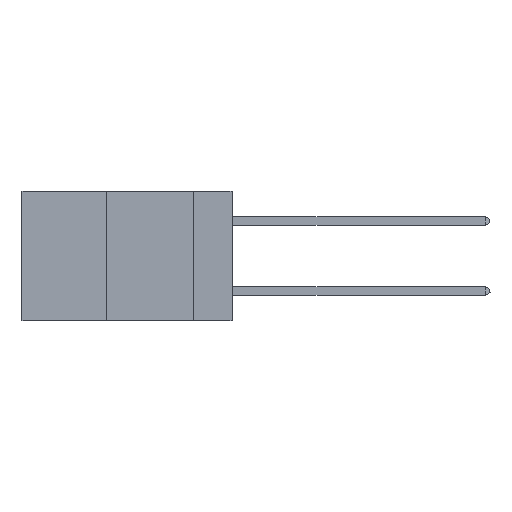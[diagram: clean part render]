
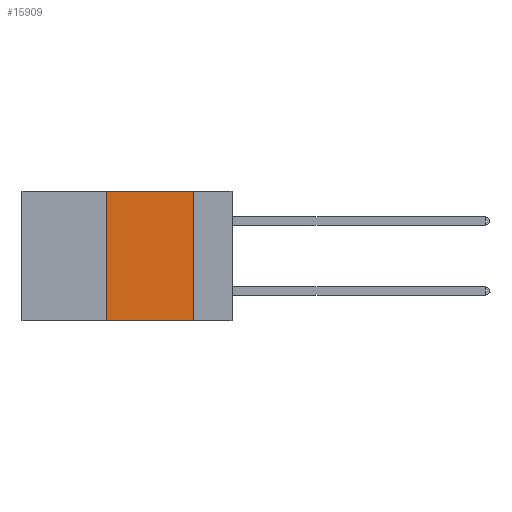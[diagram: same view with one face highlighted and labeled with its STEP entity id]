
A CAD part, left-side view. The second image highlights one B-rep face of the part: STEP entity #15909.
In plain terms, the highlighted planar face has unit normal (-1, 0, 0).
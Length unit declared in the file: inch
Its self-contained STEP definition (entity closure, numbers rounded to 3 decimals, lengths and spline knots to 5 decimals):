
#250 = VECTOR ( 'NONE', #10562, 39.37008 ) ;
#861 = ORIENTED_EDGE ( 'NONE', *, *, #14837, .F. ) ;
#1479 = EDGE_CURVE ( 'NONE', #26669, #21563, #15591, .T. ) ;
#1637 = DIRECTION ( 'NONE',  ( 0., 0., -1. ) ) ;
#2189 = CARTESIAN_POINT ( 'NONE',  ( 0., 0.6, 0. ) ) ;
#2507 = DIRECTION ( 'NONE',  ( 0., 0., 1. ) ) ;
#3303 = ORIENTED_EDGE ( 'NONE', *, *, #1479, .F. ) ;
#3799 = DIRECTION ( 'NONE',  ( 0., 0., -1. ) ) ;
#3907 = CARTESIAN_POINT ( 'NONE',  ( 0., 0.11, 0. ) ) ;
#5691 = CARTESIAN_POINT ( 'NONE',  ( 0., 0.11, 0. ) ) ;
#5751 = PLANE ( 'NONE',  #21244 ) ;
#6507 = CARTESIAN_POINT ( 'NONE',  ( 0., 0.36, 0. ) ) ;
#6688 = CARTESIAN_POINT ( 'NONE',  ( 0., 0.36, 0. ) ) ;
#7455 = LINE ( 'NONE', #2189, #250 ) ;
#7478 = EDGE_CURVE ( 'NONE', #26669, #10373, #14959, .T. ) ;
#7837 = DIRECTION ( 'NONE',  ( 1., 0., 0. ) ) ;
#10344 = LINE ( 'NONE', #5691, #27102 ) ;
#10373 = VERTEX_POINT ( 'NONE', #24117 ) ;
#10562 = DIRECTION ( 'NONE',  ( 0., -1., 0. ) ) ;
#10791 = DIRECTION ( 'NONE',  ( 0., -1., 0. ) ) ;
#12427 = CARTESIAN_POINT ( 'NONE',  ( 0., 0.36, -0.37 ) ) ;
#12949 = EDGE_CURVE ( 'NONE', #21563, #13020, #7455, .T. ) ;
#13020 = VERTEX_POINT ( 'NONE', #3907 ) ;
#14271 = FACE_OUTER_BOUND ( 'NONE', #16804, .T. ) ;
#14806 = CARTESIAN_POINT ( 'NONE',  ( 0., 0.6, -0.37 ) ) ;
#14837 = EDGE_CURVE ( 'NONE', #13020, #10373, #10344, .T. ) ;
#14959 = LINE ( 'NONE', #14806, #17218 ) ;
#15591 = LINE ( 'NONE', #6507, #26101 ) ;
#15909 = ADVANCED_FACE ( 'NONE', ( #14271 ), #5751, .F. ) ;
#16804 = EDGE_LOOP ( 'NONE', ( #861, #23595, #3303, #24495 ) ) ;
#17218 = VECTOR ( 'NONE', #10791, 39.37008 ) ;
#18066 = CARTESIAN_POINT ( 'NONE',  ( 0., 0.6, 0. ) ) ;
#21244 = AXIS2_PLACEMENT_3D ( 'NONE', #18066, #7837, #1637 ) ;
#21563 = VERTEX_POINT ( 'NONE', #6688 ) ;
#23595 = ORIENTED_EDGE ( 'NONE', *, *, #12949, .F. ) ;
#24117 = CARTESIAN_POINT ( 'NONE',  ( 0., 0.11, -0.37 ) ) ;
#24495 = ORIENTED_EDGE ( 'NONE', *, *, #7478, .T. ) ;
#26101 = VECTOR ( 'NONE', #2507, 39.37008 ) ;
#26669 = VERTEX_POINT ( 'NONE', #12427 ) ;
#27102 = VECTOR ( 'NONE', #3799, 39.37008 ) ;
